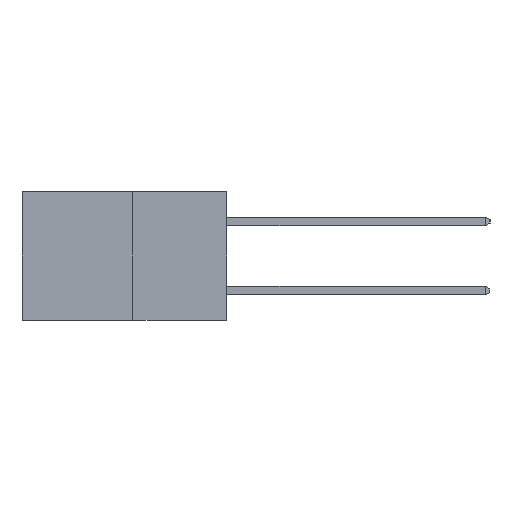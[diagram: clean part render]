
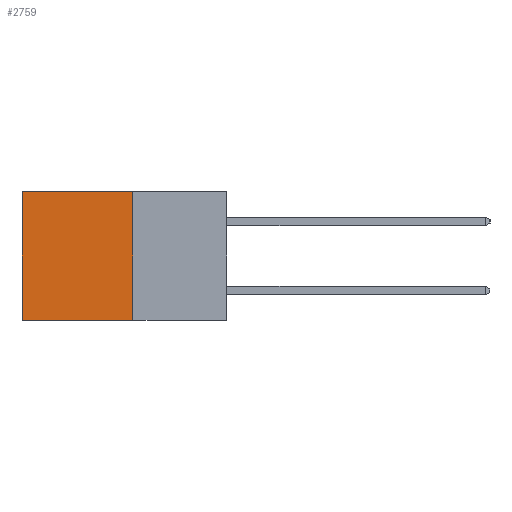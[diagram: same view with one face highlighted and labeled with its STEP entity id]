
A CAD part, left-side view. The second image highlights one B-rep face of the part: STEP entity #2759.
In plain terms, the highlighted planar face has unit normal (-1, 0, 0).
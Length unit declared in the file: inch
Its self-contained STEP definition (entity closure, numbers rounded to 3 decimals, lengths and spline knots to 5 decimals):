
#1454 = VERTEX_POINT ( 'NONE', #9168 ) ;
#1600 = LINE ( 'NONE', #6433, #3730 ) ;
#2086 = DIRECTION ( 'NONE',  ( 0., 1., 0. ) ) ;
#2183 = LINE ( 'NONE', #2372, #6809 ) ;
#2275 = CARTESIAN_POINT ( 'NONE',  ( 0.277, 0.27, -0.37 ) ) ;
#2372 = CARTESIAN_POINT ( 'NONE',  ( 0.277, 0.27, -0.37 ) ) ;
#2705 = VERTEX_POINT ( 'NONE', #4060 ) ;
#2759 = ADVANCED_FACE ( 'NONE', ( #6357 ), #11305, .F. ) ;
#2762 = CARTESIAN_POINT ( 'NONE',  ( 0.277, 0.27, 0. ) ) ;
#3400 = EDGE_CURVE ( 'NONE', #2705, #1454, #10972, .T. ) ;
#3730 = VECTOR ( 'NONE', #2086, 39.37008 ) ;
#3742 = ORIENTED_EDGE ( 'NONE', *, *, #7896, .F. ) ;
#4022 = CARTESIAN_POINT ( 'NONE',  ( 0.277, 0.27, -0.37 ) ) ;
#4060 = CARTESIAN_POINT ( 'NONE',  ( 0.277, 0.59, 0. ) ) ;
#4296 = DIRECTION ( 'NONE',  ( 0., 0., -1. ) ) ;
#4455 = ORIENTED_EDGE ( 'NONE', *, *, #8402, .T. ) ;
#5099 = VERTEX_POINT ( 'NONE', #2275 ) ;
#5383 = ORIENTED_EDGE ( 'NONE', *, *, #5402, .F. ) ;
#5402 = EDGE_CURVE ( 'NONE', #10144, #5099, #8361, .T. ) ;
#5536 = CARTESIAN_POINT ( 'NONE',  ( 0.277, 0.27, -0.37 ) ) ;
#5758 = DIRECTION ( 'NONE',  ( 0., 0., -1. ) ) ;
#5829 = DIRECTION ( 'NONE',  ( 1., 0., 0. ) ) ;
#6044 = VECTOR ( 'NONE', #4296, 39.37008 ) ;
#6357 = FACE_OUTER_BOUND ( 'NONE', #10252, .T. ) ;
#6433 = CARTESIAN_POINT ( 'NONE',  ( 0.277, 0.27, 0. ) ) ;
#6809 = VECTOR ( 'NONE', #8447, 39.37008 ) ;
#7896 = EDGE_CURVE ( 'NONE', #5099, #1454, #2183, .T. ) ;
#8361 = LINE ( 'NONE', #4022, #6044 ) ;
#8402 = EDGE_CURVE ( 'NONE', #10144, #2705, #1600, .T. ) ;
#8447 = DIRECTION ( 'NONE',  ( 0., 1., 0. ) ) ;
#8556 = CARTESIAN_POINT ( 'NONE',  ( 0.277, 0.59, -0.37 ) ) ;
#8609 = AXIS2_PLACEMENT_3D ( 'NONE', #5536, #5829, #5758 ) ;
#8848 = ORIENTED_EDGE ( 'NONE', *, *, #3400, .T. ) ;
#9168 = CARTESIAN_POINT ( 'NONE',  ( 0.277, 0.59, -0.37 ) ) ;
#10144 = VERTEX_POINT ( 'NONE', #2762 ) ;
#10252 = EDGE_LOOP ( 'NONE', ( #8848, #3742, #5383, #4455 ) ) ;
#10717 = VECTOR ( 'NONE', #10881, 39.37008 ) ;
#10881 = DIRECTION ( 'NONE',  ( 0., 0., -1. ) ) ;
#10972 = LINE ( 'NONE', #8556, #10717 ) ;
#11305 = PLANE ( 'NONE',  #8609 ) ;
